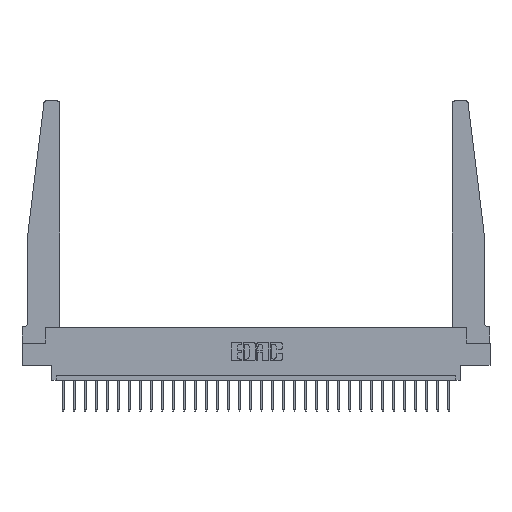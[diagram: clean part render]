
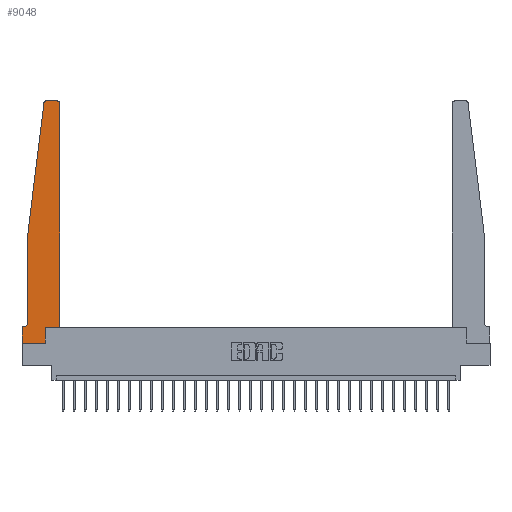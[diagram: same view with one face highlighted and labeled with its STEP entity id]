
A CAD part, top view. The second image highlights one B-rep face of the part: STEP entity #9048.
In plain terms, the highlighted planar face has unit normal (0, 0, 1).
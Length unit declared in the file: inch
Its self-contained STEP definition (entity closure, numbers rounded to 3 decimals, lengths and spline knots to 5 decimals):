
#426 = CARTESIAN_POINT ( 'NONE',  ( 0.2605, 0.18, 0.37 ) ) ;
#503 = DIRECTION ( 'NONE',  ( 0., 0., 1. ) ) ;
#855 = CARTESIAN_POINT ( 'NONE',  ( 0.25, 2.75, 0.37 ) ) ;
#1461 = VERTEX_POINT ( 'NONE', #6876 ) ;
#1477 = VERTEX_POINT ( 'NONE', #10879 ) ;
#2085 = DIRECTION ( 'NONE',  ( -1., 0., 0. ) ) ;
#2314 = CARTESIAN_POINT ( 'NONE',  ( 0.065, 1.25, 0.37 ) ) ;
#2568 = CARTESIAN_POINT ( 'NONE',  ( 0.24675, 2.72367, 0.37 ) ) ;
#2720 = LINE ( 'NONE', #27177, #11562 ) ;
#4125 = PLANE ( 'NONE',  #23680 ) ;
#4175 = ORIENTED_EDGE ( 'NONE', *, *, #10272, .T. ) ;
#4419 = CARTESIAN_POINT ( 'NONE',  ( 0.2605, 0.18, 0.37 ) ) ;
#4600 = EDGE_CURVE ( 'NONE', #13876, #24654, #20152, .T. ) ;
#5244 = EDGE_CURVE ( 'NONE', #10575, #13113, #21109, .T. ) ;
#5346 = VECTOR ( 'NONE', #15018, 39.37008 ) ;
#5882 = CARTESIAN_POINT ( 'NONE',  ( 0.2605, 0., 0.37 ) ) ;
#6134 = CARTESIAN_POINT ( 'NONE',  ( 0.425, 0.18, 0.37 ) ) ;
#6774 = CARTESIAN_POINT ( 'NONE',  ( 0., 0., 0.37 ) ) ;
#6876 = CARTESIAN_POINT ( 'NONE',  ( 0.065, 0.2375, 0.37 ) ) ;
#7606 = AXIS2_PLACEMENT_3D ( 'NONE', #13523, #503, #17868 ) ;
#8052 = CARTESIAN_POINT ( 'NONE',  ( 0.425, 2.72, 0.37 ) ) ;
#8364 = VERTEX_POINT ( 'NONE', #5882 ) ;
#8539 = VERTEX_POINT ( 'NONE', #21545 ) ;
#8684 = CARTESIAN_POINT ( 'NONE',  ( 0.065, 1.25, 0.37 ) ) ;
#8877 = VECTOR ( 'NONE', #13979, 39.37008 ) ;
#8934 = ORIENTED_EDGE ( 'NONE', *, *, #9240, .T. ) ;
#9048 = ADVANCED_FACE ( 'NONE', ( #14573 ), #4125, .T. ) ;
#9240 = EDGE_CURVE ( 'NONE', #13113, #8539, #16261, .T. ) ;
#9469 = ORIENTED_EDGE ( 'NONE', *, *, #14506, .T. ) ;
#9642 = ORIENTED_EDGE ( 'NONE', *, *, #27950, .T. ) ;
#9747 = CARTESIAN_POINT ( 'NONE',  ( 0.425, 0.18, 0.37 ) ) ;
#10145 = ORIENTED_EDGE ( 'NONE', *, *, #4600, .T. ) ;
#10272 = EDGE_CURVE ( 'NONE', #11640, #19776, #10407, .T. ) ;
#10407 = LINE ( 'NONE', #6774, #13809 ) ;
#10575 = VERTEX_POINT ( 'NONE', #21010 ) ;
#10585 = CIRCLE ( 'NONE', #7606, 0.03 ) ;
#10663 = DIRECTION ( 'NONE',  ( 0., 0., 1. ) ) ;
#10879 = CARTESIAN_POINT ( 'NONE',  ( 0.015, 0.1875, 0.37 ) ) ;
#10930 = LINE ( 'NONE', #22652, #8877 ) ;
#11110 = LINE ( 'NONE', #8684, #5346 ) ;
#11496 = ORIENTED_EDGE ( 'NONE', *, *, #22069, .T. ) ;
#11562 = VECTOR ( 'NONE', #2085, 39.37008 ) ;
#11640 = VERTEX_POINT ( 'NONE', #14472 ) ;
#11756 = CARTESIAN_POINT ( 'NONE',  ( 0.27653, 2.72, 0.37 ) ) ;
#12181 = DIRECTION ( 'NONE',  ( -1., 0., 0. ) ) ;
#12216 = VECTOR ( 'NONE', #19456, 39.37008 ) ;
#12252 = DIRECTION ( 'NONE',  ( 0., 0., -1. ) ) ;
#12943 = ORIENTED_EDGE ( 'NONE', *, *, #20438, .T. ) ;
#13113 = VERTEX_POINT ( 'NONE', #2568 ) ;
#13523 = CARTESIAN_POINT ( 'NONE',  ( 0.395, 2.72, 0.37 ) ) ;
#13809 = VECTOR ( 'NONE', #21716, 39.37008 ) ;
#13876 = VERTEX_POINT ( 'NONE', #9747 ) ;
#13979 = DIRECTION ( 'NONE',  ( 1., 0., 0. ) ) ;
#14310 = DIRECTION ( 'NONE',  ( -1., 0., 0. ) ) ;
#14416 = VECTOR ( 'NONE', #16564, 39.37008 ) ;
#14472 = CARTESIAN_POINT ( 'NONE',  ( 0., 0.1875, 0.37 ) ) ;
#14506 = EDGE_CURVE ( 'NONE', #19776, #8364, #10930, .T. ) ;
#14573 = FACE_OUTER_BOUND ( 'NONE', #16558, .T. ) ;
#15018 = DIRECTION ( 'NONE',  ( 0., -1., 0. ) ) ;
#15502 = EDGE_CURVE ( 'NONE', #17619, #13876, #24060, .T. ) ;
#15661 = LINE ( 'NONE', #855, #20713 ) ;
#16070 = ORIENTED_EDGE ( 'NONE', *, *, #15502, .T. ) ;
#16158 = VECTOR ( 'NONE', #22208, 39.37008 ) ;
#16261 = LINE ( 'NONE', #2314, #12216 ) ;
#16532 = CARTESIAN_POINT ( 'NONE',  ( 0.395, 2.75, 0.37 ) ) ;
#16558 = EDGE_LOOP ( 'NONE', ( #11496, #27596, #8934, #9642, #25173, #25639, #4175, #9469, #25556, #16070, #10145, #12943 ) ) ;
#16564 = DIRECTION ( 'NONE',  ( 0., 1., 0. ) ) ;
#16766 = VERTEX_POINT ( 'NONE', #16532 ) ;
#16905 = DIRECTION ( 'NONE',  ( 1., 0., 0. ) ) ;
#17619 = VERTEX_POINT ( 'NONE', #4419 ) ;
#17868 = DIRECTION ( 'NONE',  ( 1., 0., 0. ) ) ;
#18238 = DIRECTION ( 'NONE',  ( 1., 0., 0. ) ) ;
#19456 = DIRECTION ( 'NONE',  ( -0.122, -0.992, 0. ) ) ;
#19776 = VERTEX_POINT ( 'NONE', #24536 ) ;
#19848 = CARTESIAN_POINT ( 'NONE',  ( 0.425, 0.18, 0.37 ) ) ;
#20152 = LINE ( 'NONE', #6134, #14416 ) ;
#20438 = EDGE_CURVE ( 'NONE', #24654, #16766, #10585, .T. ) ;
#20713 = VECTOR ( 'NONE', #12181, 39.37008 ) ;
#20792 = EDGE_CURVE ( 'NONE', #1461, #1477, #22400, .T. ) ;
#20899 = AXIS2_PLACEMENT_3D ( 'NONE', #11756, #26859, #18238 ) ;
#21010 = CARTESIAN_POINT ( 'NONE',  ( 0.27653, 2.75, 0.37 ) ) ;
#21109 = CIRCLE ( 'NONE', #20899, 0.03 ) ;
#21508 = CARTESIAN_POINT ( 'NONE',  ( 0., 0.1875, 0.37 ) ) ;
#21545 = CARTESIAN_POINT ( 'NONE',  ( 0.065, 1.25, 0.37 ) ) ;
#21716 = DIRECTION ( 'NONE',  ( 0., -1., 0. ) ) ;
#21876 = LINE ( 'NONE', #426, #16158 ) ;
#21897 = DIRECTION ( 'NONE',  ( 1., 0., 0. ) ) ;
#22069 = EDGE_CURVE ( 'NONE', #16766, #10575, #15661, .T. ) ;
#22208 = DIRECTION ( 'NONE',  ( 0., 1., 0. ) ) ;
#22400 = CIRCLE ( 'NONE', #27719, 0.05 ) ;
#22652 = CARTESIAN_POINT ( 'NONE',  ( 0., 0., 0.37 ) ) ;
#22726 = EDGE_CURVE ( 'NONE', #1477, #11640, #2720, .T. ) ;
#22800 = CARTESIAN_POINT ( 'NONE',  ( 0.015, 0.2375, 0.37 ) ) ;
#23680 = AXIS2_PLACEMENT_3D ( 'NONE', #21508, #10663, #16905 ) ;
#23723 = VECTOR ( 'NONE', #21897, 39.37008 ) ;
#24060 = LINE ( 'NONE', #19848, #23723 ) ;
#24536 = CARTESIAN_POINT ( 'NONE',  ( 0., 0., 0.37 ) ) ;
#24654 = VERTEX_POINT ( 'NONE', #8052 ) ;
#24878 = EDGE_CURVE ( 'NONE', #8364, #17619, #21876, .T. ) ;
#25173 = ORIENTED_EDGE ( 'NONE', *, *, #20792, .T. ) ;
#25556 = ORIENTED_EDGE ( 'NONE', *, *, #24878, .T. ) ;
#25639 = ORIENTED_EDGE ( 'NONE', *, *, #22726, .T. ) ;
#26859 = DIRECTION ( 'NONE',  ( 0., 0., 1. ) ) ;
#27177 = CARTESIAN_POINT ( 'NONE',  ( 0.065, 0.1875, 0.37 ) ) ;
#27596 = ORIENTED_EDGE ( 'NONE', *, *, #5244, .T. ) ;
#27719 = AXIS2_PLACEMENT_3D ( 'NONE', #22800, #12252, #14310 ) ;
#27950 = EDGE_CURVE ( 'NONE', #8539, #1461, #11110, .T. ) ;
